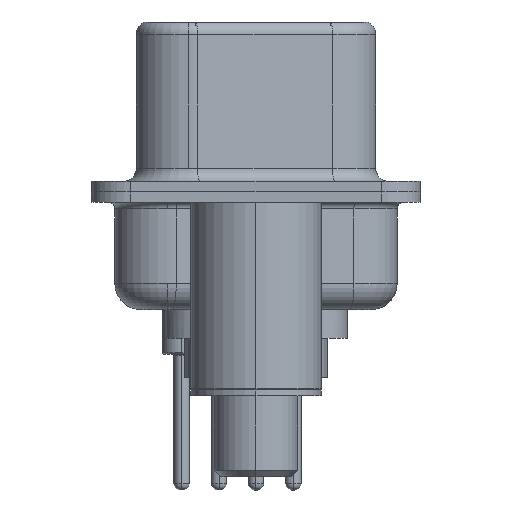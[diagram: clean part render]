
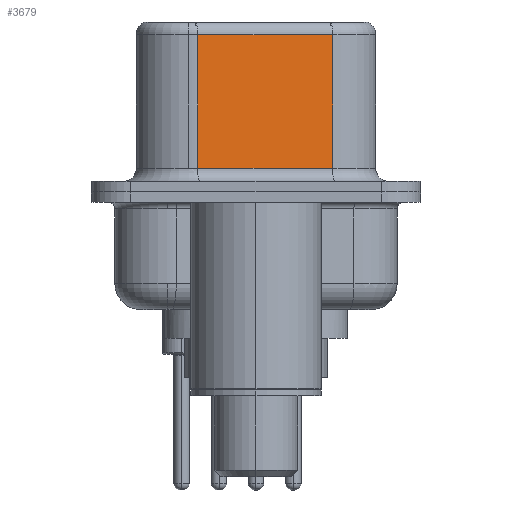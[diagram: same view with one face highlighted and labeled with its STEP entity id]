
A CAD part, left-side view. The second image highlights one B-rep face of the part: STEP entity #3679.
In plain terms, the highlighted planar face has unit normal (-0.985, -0.174, 0).
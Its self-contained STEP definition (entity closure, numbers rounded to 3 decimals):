
#186 = DIRECTION ( 'NONE',  ( 0.985, 0.174, 0. ) ) ;
#331 = FACE_OUTER_BOUND ( 'NONE', #16598, .T. ) ;
#447 = VECTOR ( 'NONE', #17293, 1000. ) ;
#648 = DIRECTION ( 'NONE',  ( -0.174, 0.985, 0. ) ) ;
#1041 = LINE ( 'NONE', #19263, #10487 ) ;
#3679 = ADVANCED_FACE ( 'NONE', ( #331 ), #9594, .F. ) ;
#3854 = ORIENTED_EDGE ( 'NONE', *, *, #21446, .T. ) ;
#4459 = CARTESIAN_POINT ( 'NONE',  ( 4.58, -2.927, 6.02 ) ) ;
#5176 = CARTESIAN_POINT ( 'NONE',  ( 4.58, -2.927, 6.52 ) ) ;
#6146 = ORIENTED_EDGE ( 'NONE', *, *, #22552, .T. ) ;
#7700 = CARTESIAN_POINT ( 'NONE',  ( 4.58, -2.927, 6.52 ) ) ;
#8164 = VECTOR ( 'NONE', #8903, 1000. ) ;
#8903 = DIRECTION ( 'NONE',  ( 0., 0., -1. ) ) ;
#9072 = EDGE_CURVE ( 'NONE', #24575, #16965, #18344, .T. ) ;
#9594 = PLANE ( 'NONE',  #15455 ) ;
#10487 = VECTOR ( 'NONE', #11555, 1000. ) ;
#10693 = CARTESIAN_POINT ( 'NONE',  ( 4.58, -2.927, 6.02 ) ) ;
#11555 = DIRECTION ( 'NONE',  ( 0.174, -0.985, 0. ) ) ;
#13453 = DIRECTION ( 'NONE',  ( -0.174, 0.985, 0. ) ) ;
#13628 = ORIENTED_EDGE ( 'NONE', *, *, #9072, .F. ) ;
#14478 = LINE ( 'NONE', #4459, #18933 ) ;
#15151 = ORIENTED_EDGE ( 'NONE', *, *, #22548, .T. ) ;
#15455 = AXIS2_PLACEMENT_3D ( 'NONE', #7700, #186, #13453 ) ;
#15658 = LINE ( 'NONE', #23068, #447 ) ;
#15814 = VERTEX_POINT ( 'NONE', #22466 ) ;
#16598 = EDGE_LOOP ( 'NONE', ( #13628, #3854, #6146, #15151 ) ) ;
#16965 = VERTEX_POINT ( 'NONE', #24495 ) ;
#17293 = DIRECTION ( 'NONE',  ( 0., 0., -1. ) ) ;
#18344 = LINE ( 'NONE', #5176, #8164 ) ;
#18933 = VECTOR ( 'NONE', #648, 1000. ) ;
#19263 = CARTESIAN_POINT ( 'NONE',  ( 4.58, -2.927, 0.9 ) ) ;
#20056 = VERTEX_POINT ( 'NONE', #24295 ) ;
#21446 = EDGE_CURVE ( 'NONE', #24575, #20056, #14478, .T. ) ;
#22466 = CARTESIAN_POINT ( 'NONE',  ( 3.67, 2.233, 0.9 ) ) ;
#22548 = EDGE_CURVE ( 'NONE', #15814, #16965, #1041, .T. ) ;
#22552 = EDGE_CURVE ( 'NONE', #20056, #15814, #15658, .T. ) ;
#23068 = CARTESIAN_POINT ( 'NONE',  ( 3.67, 2.233, 6.52 ) ) ;
#24295 = CARTESIAN_POINT ( 'NONE',  ( 3.67, 2.233, 6.02 ) ) ;
#24495 = CARTESIAN_POINT ( 'NONE',  ( 4.58, -2.927, 0.9 ) ) ;
#24575 = VERTEX_POINT ( 'NONE', #10693 ) ;
